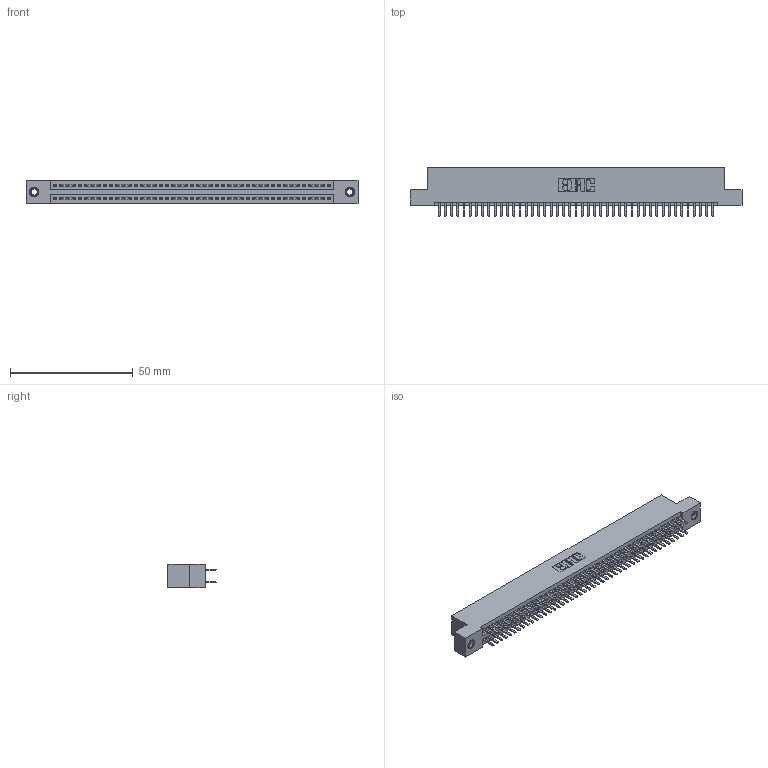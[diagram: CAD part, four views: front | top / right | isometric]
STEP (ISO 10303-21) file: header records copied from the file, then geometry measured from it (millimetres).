
FILE_DESCRIPTION (( 'STEP AP203' ), '1' );
FILE_NAME ('395-090-520-207.STEP', '2019-10-25T15:39:47', ( '' ), ( '' ), 'SwSTEP 2.0', 'SolidWorks 2016', '' );
FILE_SCHEMA (( 'CONFIG_CONTROL_DESIGN' ));
Length unit declared in the file: inch
Products named in the file (4): 345 Part_Flush Mounting Lugs - 0.156 Dia-TI; 345-292-001_345-293-120; 345-250-001_345-250-005-103; 395-090-520-207
Assembly tree (93 placements, depth 2):
  395-090-520-207
    345 Part_Flush Mounting Lugs - 0.156 Dia-TI
    345-292-001_345-293-120  x90
    345-250-001_345-250-005-103  x2
Bounding box: 135.51 x 19.68 x 9.4 mm (x, y, z)
Volume: 13138.2 mm3; surface area: 19422.4 mm2
Topology: 93 solids, 93 shells, 5046 faces, 14607 edges, 9490 vertices
Faces by surface type: plane 3262, cylinder 1768, cone 12, torus 4
Entity records: 36204 total; most frequent: CARTESIAN_POINT 6059, ORIENTED_EDGE 5974, DIRECTION 5353, EDGE_CURVE 2987, LINE 2651, VECTOR 2651, VERTEX_POINT 1984, AXIS2_PLACEMENT_3D 1351
